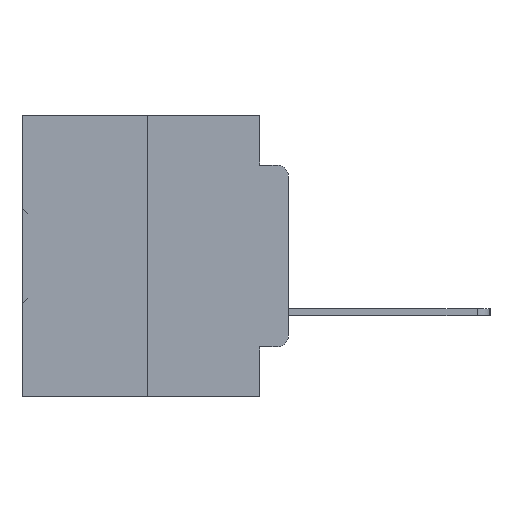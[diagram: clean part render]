
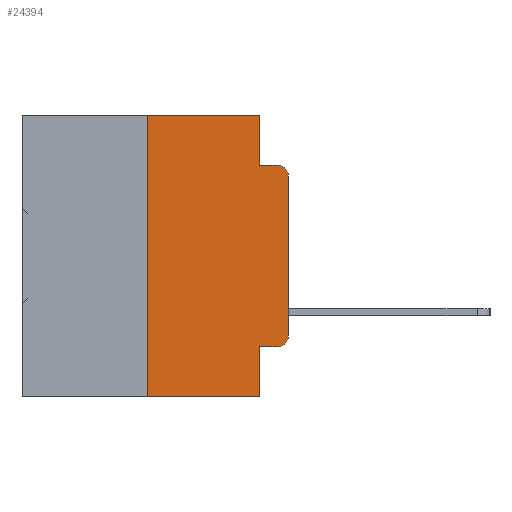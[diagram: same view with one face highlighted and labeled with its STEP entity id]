
A CAD part, left-side view. The second image highlights one B-rep face of the part: STEP entity #24394.
In plain terms, the highlighted planar face has unit normal (-1, 0, 0).
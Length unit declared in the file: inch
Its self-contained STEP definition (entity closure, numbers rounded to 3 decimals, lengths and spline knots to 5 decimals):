
#318 = PLANE ( 'NONE',  #23862 ) ;
#809 = LINE ( 'NONE', #17074, #22264 ) ;
#945 = DIRECTION ( 'NONE',  ( 0., 0., -1. ) ) ;
#1969 = CARTESIAN_POINT ( 'NONE',  ( 0., 0.02, -0.0885 ) ) ;
#2052 = LINE ( 'NONE', #4428, #16669 ) ;
#2877 = ORIENTED_EDGE ( 'NONE', *, *, #13203, .T. ) ;
#3243 = DIRECTION ( 'NONE',  ( 0., 0., -1. ) ) ;
#3280 = VERTEX_POINT ( 'NONE', #19411 ) ;
#3416 = EDGE_CURVE ( 'NONE', #3280, #17209, #4423, .T. ) ;
#3539 = DIRECTION ( 'NONE',  ( 0., 0., -1. ) ) ;
#4081 = CARTESIAN_POINT ( 'NONE',  ( 0., 0., -0.3915 ) ) ;
#4161 = EDGE_CURVE ( 'NONE', #6870, #14944, #20803, .T. ) ;
#4423 = LINE ( 'NONE', #23234, #31770 ) ;
#4428 = CARTESIAN_POINT ( 'NONE',  ( 0., 0.473, 0. ) ) ;
#4488 = ORIENTED_EDGE ( 'NONE', *, *, #11350, .F. ) ;
#4638 = CARTESIAN_POINT ( 'NONE',  ( 0., 0.051, -0.5 ) ) ;
#5114 = VECTOR ( 'NONE', #3539, 39.37008 ) ;
#5716 = DIRECTION ( 'NONE',  ( 0., -1., 0. ) ) ;
#6463 = CARTESIAN_POINT ( 'NONE',  ( 0., 0.473, -0.5 ) ) ;
#6737 = ORIENTED_EDGE ( 'NONE', *, *, #35341, .F. ) ;
#6870 = VERTEX_POINT ( 'NONE', #31035 ) ;
#7314 = EDGE_CURVE ( 'NONE', #25046, #17209, #27245, .T. ) ;
#7887 = ORIENTED_EDGE ( 'NONE', *, *, #3416, .F. ) ;
#8472 = DIRECTION ( 'NONE',  ( 0., 0., 1. ) ) ;
#8539 = LINE ( 'NONE', #9961, #23208 ) ;
#8574 = CARTESIAN_POINT ( 'NONE',  ( 0., 0.02, -0.3915 ) ) ;
#8854 = ORIENTED_EDGE ( 'NONE', *, *, #4161, .T. ) ;
#8939 = CARTESIAN_POINT ( 'NONE',  ( 0., 0.473, 0. ) ) ;
#9374 = DIRECTION ( 'NONE',  ( 0., -1., 0. ) ) ;
#9395 = VECTOR ( 'NONE', #32093, 39.37008 ) ;
#9961 = CARTESIAN_POINT ( 'NONE',  ( 0., 0.051, -0.4115 ) ) ;
#10328 = LINE ( 'NONE', #30264, #9395 ) ;
#11350 = EDGE_CURVE ( 'NONE', #14761, #15760, #2052, .T. ) ;
#11551 = DIRECTION ( 'NONE',  ( 0., 0., -1. ) ) ;
#11799 = ORIENTED_EDGE ( 'NONE', *, *, #33451, .F. ) ;
#12110 = CARTESIAN_POINT ( 'NONE',  ( 0., 0.25, 0. ) ) ;
#12208 = CARTESIAN_POINT ( 'NONE',  ( 0., 0.051, 0. ) ) ;
#13203 = EDGE_CURVE ( 'NONE', #14944, #25046, #36016, .T. ) ;
#13785 = LINE ( 'NONE', #12208, #5114 ) ;
#14761 = VERTEX_POINT ( 'NONE', #12110 ) ;
#14944 = VERTEX_POINT ( 'NONE', #4081 ) ;
#15372 = VERTEX_POINT ( 'NONE', #4638 ) ;
#15760 = VERTEX_POINT ( 'NONE', #26538 ) ;
#15885 = EDGE_CURVE ( 'NONE', #26509, #6870, #8539, .T. ) ;
#16669 = VECTOR ( 'NONE', #27747, 39.37008 ) ;
#17040 = VERTEX_POINT ( 'NONE', #33198 ) ;
#17074 = CARTESIAN_POINT ( 'NONE',  ( 0., 0.25, 0. ) ) ;
#17209 = VERTEX_POINT ( 'NONE', #1969 ) ;
#17963 = ORIENTED_EDGE ( 'NONE', *, *, #7314, .T. ) ;
#18445 = DIRECTION ( 'NONE',  ( -1., 0., 0. ) ) ;
#18878 = EDGE_CURVE ( 'NONE', #17040, #15372, #30858, .T. ) ;
#19411 = CARTESIAN_POINT ( 'NONE',  ( 0., 0.051, -0.0885 ) ) ;
#19523 = DIRECTION ( 'NONE',  ( 0., 0., 1. ) ) ;
#20743 = DIRECTION ( 'NONE',  ( 1., 0., 0. ) ) ;
#20803 = CIRCLE ( 'NONE', #35003, 0.02 ) ;
#21264 = AXIS2_PLACEMENT_3D ( 'NONE', #35782, #18445, #945 ) ;
#22264 = VECTOR ( 'NONE', #8472, 39.37008 ) ;
#22356 = ORIENTED_EDGE ( 'NONE', *, *, #23739, .F. ) ;
#23208 = VECTOR ( 'NONE', #30350, 39.37008 ) ;
#23234 = CARTESIAN_POINT ( 'NONE',  ( 0., 0.051, -0.0885 ) ) ;
#23739 = EDGE_CURVE ( 'NONE', #26509, #15372, #10328, .T. ) ;
#23862 = AXIS2_PLACEMENT_3D ( 'NONE', #8939, #20743, #3243 ) ;
#24394 = ADVANCED_FACE ( 'NONE', ( #33070 ), #318, .F. ) ;
#25046 = VERTEX_POINT ( 'NONE', #29307 ) ;
#26509 = VERTEX_POINT ( 'NONE', #27934 ) ;
#26538 = CARTESIAN_POINT ( 'NONE',  ( 0., 0.051, 0. ) ) ;
#26866 = ORIENTED_EDGE ( 'NONE', *, *, #18878, .T. ) ;
#27245 = CIRCLE ( 'NONE', #21264, 0.02 ) ;
#27443 = VECTOR ( 'NONE', #19523, 39.37008 ) ;
#27511 = EDGE_LOOP ( 'NONE', ( #2877, #17963, #7887, #6737, #4488, #11799, #26866, #22356, #36026, #8854 ) ) ;
#27747 = DIRECTION ( 'NONE',  ( 0., -1., 0. ) ) ;
#27934 = CARTESIAN_POINT ( 'NONE',  ( 0., 0.051, -0.4115 ) ) ;
#28985 = DIRECTION ( 'NONE',  ( -1., 0., 0. ) ) ;
#29307 = CARTESIAN_POINT ( 'NONE',  ( 0., 0., -0.1085 ) ) ;
#29961 = VECTOR ( 'NONE', #9374, 39.37008 ) ;
#30264 = CARTESIAN_POINT ( 'NONE',  ( 0., 0.051, 0. ) ) ;
#30350 = DIRECTION ( 'NONE',  ( 0., -1., 0. ) ) ;
#30858 = LINE ( 'NONE', #6463, #29961 ) ;
#31035 = CARTESIAN_POINT ( 'NONE',  ( 0., 0.02, -0.4115 ) ) ;
#31210 = CARTESIAN_POINT ( 'NONE',  ( 0., 0., 0. ) ) ;
#31770 = VECTOR ( 'NONE', #5716, 39.37008 ) ;
#32093 = DIRECTION ( 'NONE',  ( 0., 0., -1. ) ) ;
#33070 = FACE_OUTER_BOUND ( 'NONE', #27511, .T. ) ;
#33198 = CARTESIAN_POINT ( 'NONE',  ( 0., 0.25, -0.5 ) ) ;
#33451 = EDGE_CURVE ( 'NONE', #17040, #14761, #809, .T. ) ;
#35003 = AXIS2_PLACEMENT_3D ( 'NONE', #8574, #28985, #11551 ) ;
#35341 = EDGE_CURVE ( 'NONE', #15760, #3280, #13785, .T. ) ;
#35782 = CARTESIAN_POINT ( 'NONE',  ( 0., 0.02, -0.1085 ) ) ;
#36016 = LINE ( 'NONE', #31210, #27443 ) ;
#36026 = ORIENTED_EDGE ( 'NONE', *, *, #15885, .T. ) ;
